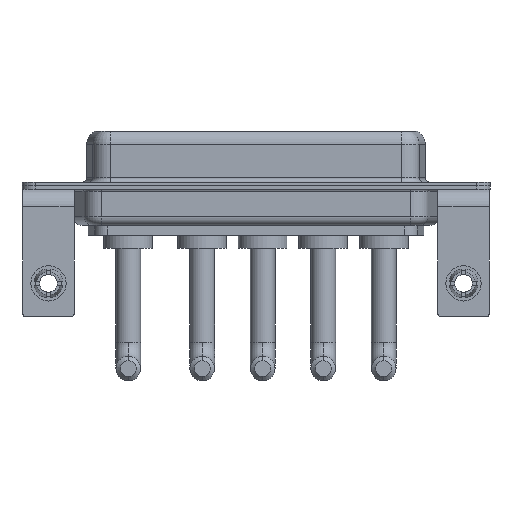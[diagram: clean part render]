
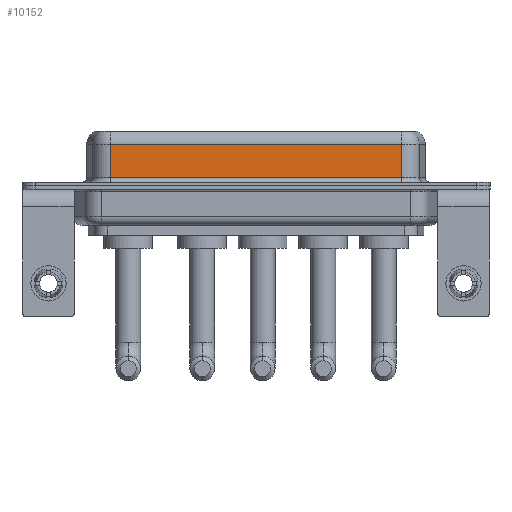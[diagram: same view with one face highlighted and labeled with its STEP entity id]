
A CAD part, front view. The second image highlights one B-rep face of the part: STEP entity #10152.
In plain terms, the highlighted planar face has unit normal (0, -1, 0).
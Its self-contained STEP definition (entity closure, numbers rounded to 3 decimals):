
#208 = AXIS2_PLACEMENT_3D ( 'NONE', #4410, #13702, #3256 ) ;
#659 = VECTOR ( 'NONE', #4624, 1000. ) ;
#1952 = CARTESIAN_POINT ( 'NONE',  ( 7.013, -3.95, 0.9 ) ) ;
#2172 = CARTESIAN_POINT ( 'NONE',  ( 40.037, -3.95, 0.9 ) ) ;
#3191 = CARTESIAN_POINT ( 'NONE',  ( 40.037, -3.95, 0.9 ) ) ;
#3256 = DIRECTION ( 'NONE',  ( 0., 0., 1. ) ) ;
#3327 = LINE ( 'NONE', #11487, #659 ) ;
#3715 = ORIENTED_EDGE ( 'NONE', *, *, #12310, .T. ) ;
#3754 = LINE ( 'NONE', #4908, #9215 ) ;
#3856 = EDGE_CURVE ( 'NONE', #13816, #13858, #3754, .T. ) ;
#3987 = ORIENTED_EDGE ( 'NONE', *, *, #9863, .F. ) ;
#4292 = VERTEX_POINT ( 'NONE', #14862 ) ;
#4358 = EDGE_CURVE ( 'NONE', #13858, #12264, #10057, .T. ) ;
#4410 = CARTESIAN_POINT ( 'NONE',  ( 40.037, -3.95, 6.4 ) ) ;
#4624 = DIRECTION ( 'NONE',  ( -1., 0., 0. ) ) ;
#4908 = CARTESIAN_POINT ( 'NONE',  ( 7.013, -3.95, 6.4 ) ) ;
#5562 = ORIENTED_EDGE ( 'NONE', *, *, #3856, .T. ) ;
#5643 = EDGE_LOOP ( 'NONE', ( #3987, #3715, #5562, #7392 ) ) ;
#7303 = VECTOR ( 'NONE', #11791, 1000. ) ;
#7392 = ORIENTED_EDGE ( 'NONE', *, *, #4358, .T. ) ;
#8282 = LINE ( 'NONE', #12935, #7303 ) ;
#8987 = VECTOR ( 'NONE', #14932, 1000. ) ;
#9215 = VECTOR ( 'NONE', #9549, 1000. ) ;
#9549 = DIRECTION ( 'NONE',  ( 0., 0., -1. ) ) ;
#9863 = EDGE_CURVE ( 'NONE', #4292, #12264, #8282, .T. ) ;
#10057 = LINE ( 'NONE', #3191, #8987 ) ;
#10152 = ADVANCED_FACE ( 'NONE', ( #14857 ), #14713, .F. ) ;
#11487 = CARTESIAN_POINT ( 'NONE',  ( 40.037, -3.95, 4.65 ) ) ;
#11791 = DIRECTION ( 'NONE',  ( 0., 0., -1. ) ) ;
#12264 = VERTEX_POINT ( 'NONE', #2172 ) ;
#12310 = EDGE_CURVE ( 'NONE', #4292, #13816, #3327, .T. ) ;
#12324 = CARTESIAN_POINT ( 'NONE',  ( 7.013, -3.95, 4.65 ) ) ;
#12935 = CARTESIAN_POINT ( 'NONE',  ( 40.037, -3.95, 6.4 ) ) ;
#13702 = DIRECTION ( 'NONE',  ( 0., 1., 0. ) ) ;
#13816 = VERTEX_POINT ( 'NONE', #12324 ) ;
#13858 = VERTEX_POINT ( 'NONE', #1952 ) ;
#14713 = PLANE ( 'NONE',  #208 ) ;
#14857 = FACE_OUTER_BOUND ( 'NONE', #5643, .T. ) ;
#14862 = CARTESIAN_POINT ( 'NONE',  ( 40.037, -3.95, 4.65 ) ) ;
#14932 = DIRECTION ( 'NONE',  ( 1., 0., 0. ) ) ;
